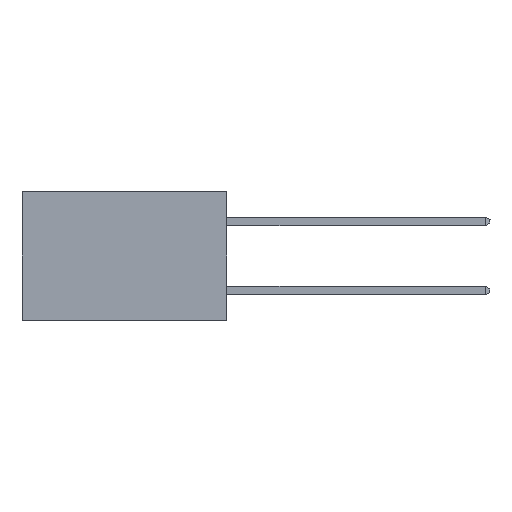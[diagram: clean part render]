
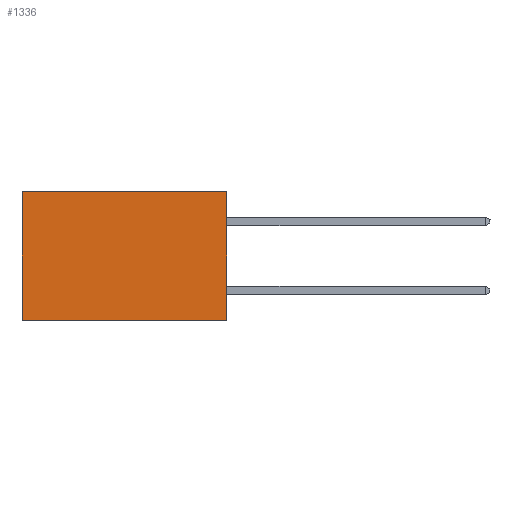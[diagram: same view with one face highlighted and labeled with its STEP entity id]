
A CAD part, left-side view. The second image highlights one B-rep face of the part: STEP entity #1336.
In plain terms, the highlighted planar face has unit normal (-1, 0, 0).
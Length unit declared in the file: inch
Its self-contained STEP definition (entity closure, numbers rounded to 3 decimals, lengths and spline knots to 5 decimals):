
#478 = EDGE_CURVE ( 'NONE', #9031, #6668, #11729, .T. ) ;
#959 = EDGE_CURVE ( 'NONE', #12342, #6668, #8947, .T. ) ;
#1336 = ADVANCED_FACE ( 'NONE', ( #8505 ), #3668, .F. ) ;
#2046 = CARTESIAN_POINT ( 'NONE',  ( 0.277, 0.59, -0.37 ) ) ;
#2535 = LINE ( 'NONE', #7737, #7209 ) ;
#3258 = CARTESIAN_POINT ( 'NONE',  ( 0.277, 0., -0.37 ) ) ;
#3573 = CARTESIAN_POINT ( 'NONE',  ( 0.277, 0.59, 0. ) ) ;
#3668 = PLANE ( 'NONE',  #4369 ) ;
#3959 = VECTOR ( 'NONE', #8624, 39.37008 ) ;
#4216 = DIRECTION ( 'NONE',  ( 0., 0., -1. ) ) ;
#4369 = AXIS2_PLACEMENT_3D ( 'NONE', #5437, #6157, #4216 ) ;
#4822 = CARTESIAN_POINT ( 'NONE',  ( 0.277, 0., -0.37 ) ) ;
#4945 = CARTESIAN_POINT ( 'NONE',  ( 0.277, 0.59, -0.37 ) ) ;
#5437 = CARTESIAN_POINT ( 'NONE',  ( 0.277, 0., -0.37 ) ) ;
#6061 = VECTOR ( 'NONE', #7888, 39.37008 ) ;
#6157 = DIRECTION ( 'NONE',  ( 1., 0., 0. ) ) ;
#6668 = VERTEX_POINT ( 'NONE', #4945 ) ;
#7067 = VECTOR ( 'NONE', #8415, 39.37008 ) ;
#7209 = VECTOR ( 'NONE', #7674, 39.37008 ) ;
#7674 = DIRECTION ( 'NONE',  ( 0., 1., 0. ) ) ;
#7737 = CARTESIAN_POINT ( 'NONE',  ( 0.277, 0., 0. ) ) ;
#7888 = DIRECTION ( 'NONE',  ( 0., 1., 0. ) ) ;
#8124 = EDGE_LOOP ( 'NONE', ( #10141, #10128, #10168, #9833 ) ) ;
#8415 = DIRECTION ( 'NONE',  ( 0., 0., -1. ) ) ;
#8441 = CARTESIAN_POINT ( 'NONE',  ( 0.277, 0., -0.37 ) ) ;
#8505 = FACE_OUTER_BOUND ( 'NONE', #8124, .T. ) ;
#8624 = DIRECTION ( 'NONE',  ( 0., 0., -1. ) ) ;
#8727 = EDGE_CURVE ( 'NONE', #11520, #12342, #2535, .T. ) ;
#8947 = LINE ( 'NONE', #2046, #3959 ) ;
#9031 = VERTEX_POINT ( 'NONE', #3258 ) ;
#9608 = CARTESIAN_POINT ( 'NONE',  ( 0.277, 0., 0. ) ) ;
#9833 = ORIENTED_EDGE ( 'NONE', *, *, #8727, .T. ) ;
#10041 = EDGE_CURVE ( 'NONE', #11520, #9031, #12184, .T. ) ;
#10128 = ORIENTED_EDGE ( 'NONE', *, *, #478, .F. ) ;
#10141 = ORIENTED_EDGE ( 'NONE', *, *, #959, .T. ) ;
#10168 = ORIENTED_EDGE ( 'NONE', *, *, #10041, .F. ) ;
#11520 = VERTEX_POINT ( 'NONE', #9608 ) ;
#11729 = LINE ( 'NONE', #4822, #6061 ) ;
#12184 = LINE ( 'NONE', #8441, #7067 ) ;
#12342 = VERTEX_POINT ( 'NONE', #3573 ) ;
